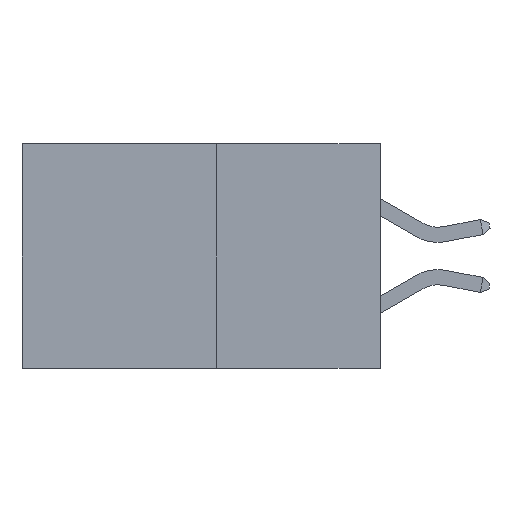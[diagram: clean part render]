
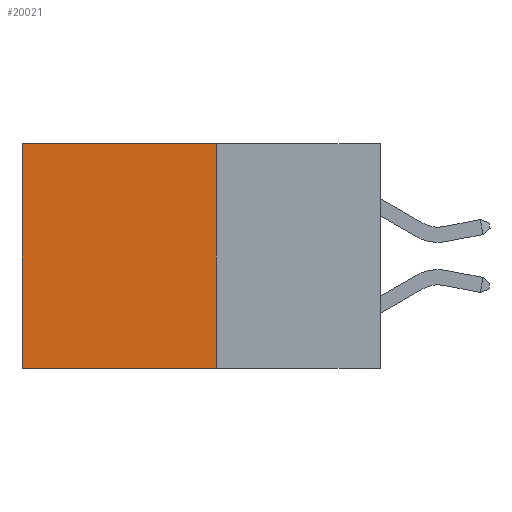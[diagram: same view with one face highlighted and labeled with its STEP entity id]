
A CAD part, left-side view. The second image highlights one B-rep face of the part: STEP entity #20021.
In plain terms, the highlighted planar face has unit normal (-1, 0, 0).
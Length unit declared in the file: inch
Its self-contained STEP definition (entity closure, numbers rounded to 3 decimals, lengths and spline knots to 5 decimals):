
#117 = VECTOR ( 'NONE', #14464, 39.37008 ) ;
#259 = CARTESIAN_POINT ( 'NONE',  ( 0.277, 0.27, -0.37 ) ) ;
#1657 = CARTESIAN_POINT ( 'NONE',  ( 0.277, 0.59, -0.37 ) ) ;
#1975 = AXIS2_PLACEMENT_3D ( 'NONE', #10512, #12191, #2146 ) ;
#2146 = DIRECTION ( 'NONE',  ( 0., 0., -1. ) ) ;
#2681 = CARTESIAN_POINT ( 'NONE',  ( 0.277, 0.27, 0. ) ) ;
#3934 = LINE ( 'NONE', #2681, #117 ) ;
#4262 = DIRECTION ( 'NONE',  ( 0., 0., -1. ) ) ;
#4322 = DIRECTION ( 'NONE',  ( 0., 0., -1. ) ) ;
#4833 = VECTOR ( 'NONE', #4322, 39.37008 ) ;
#4906 = CARTESIAN_POINT ( 'NONE',  ( 0.277, 0.27, -0.37 ) ) ;
#4946 = LINE ( 'NONE', #4906, #13402 ) ;
#4992 = CARTESIAN_POINT ( 'NONE',  ( 0.277, 0.27, -0.37 ) ) ;
#5287 = ORIENTED_EDGE ( 'NONE', *, *, #16382, .T. ) ;
#5626 = CARTESIAN_POINT ( 'NONE',  ( 0.277, 0.59, 0. ) ) ;
#5913 = LINE ( 'NONE', #11052, #4833 ) ;
#6641 = DIRECTION ( 'NONE',  ( 0., 1., 0. ) ) ;
#7282 = EDGE_CURVE ( 'NONE', #14101, #21287, #9001, .T. ) ;
#7405 = FACE_OUTER_BOUND ( 'NONE', #11299, .T. ) ;
#8490 = VERTEX_POINT ( 'NONE', #1657 ) ;
#8824 = PLANE ( 'NONE',  #1975 ) ;
#9001 = LINE ( 'NONE', #4992, #12406 ) ;
#9637 = CARTESIAN_POINT ( 'NONE',  ( 0.277, 0.27, 0. ) ) ;
#10512 = CARTESIAN_POINT ( 'NONE',  ( 0.277, 0.27, -0.37 ) ) ;
#11052 = CARTESIAN_POINT ( 'NONE',  ( 0.277, 0.59, -0.37 ) ) ;
#11299 = EDGE_LOOP ( 'NONE', ( #13093, #14927, #17354, #5287 ) ) ;
#12191 = DIRECTION ( 'NONE',  ( 1., 0., 0. ) ) ;
#12406 = VECTOR ( 'NONE', #4262, 39.37008 ) ;
#13093 = ORIENTED_EDGE ( 'NONE', *, *, #13511, .T. ) ;
#13402 = VECTOR ( 'NONE', #6641, 39.37008 ) ;
#13511 = EDGE_CURVE ( 'NONE', #18204, #8490, #5913, .T. ) ;
#14101 = VERTEX_POINT ( 'NONE', #9637 ) ;
#14464 = DIRECTION ( 'NONE',  ( 0., 1., 0. ) ) ;
#14927 = ORIENTED_EDGE ( 'NONE', *, *, #17111, .F. ) ;
#16382 = EDGE_CURVE ( 'NONE', #14101, #18204, #3934, .T. ) ;
#17111 = EDGE_CURVE ( 'NONE', #21287, #8490, #4946, .T. ) ;
#17354 = ORIENTED_EDGE ( 'NONE', *, *, #7282, .F. ) ;
#18204 = VERTEX_POINT ( 'NONE', #5626 ) ;
#20021 = ADVANCED_FACE ( 'NONE', ( #7405 ), #8824, .F. ) ;
#21287 = VERTEX_POINT ( 'NONE', #259 ) ;
